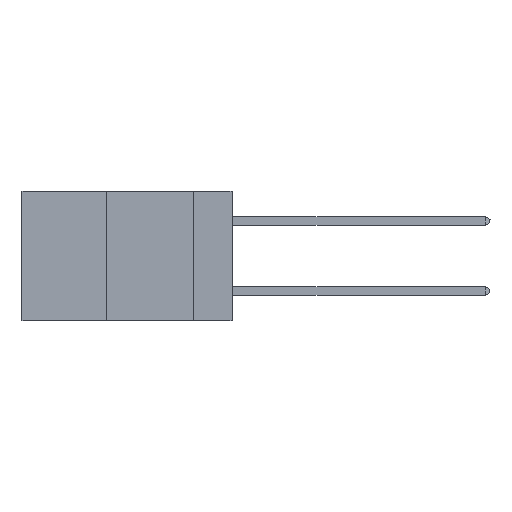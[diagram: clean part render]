
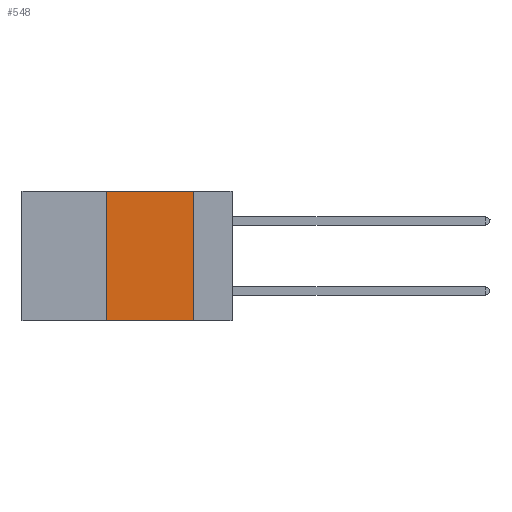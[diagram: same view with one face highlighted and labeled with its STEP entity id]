
A CAD part, left-side view. The second image highlights one B-rep face of the part: STEP entity #548.
In plain terms, the highlighted planar face has unit normal (-1, 0, 0).
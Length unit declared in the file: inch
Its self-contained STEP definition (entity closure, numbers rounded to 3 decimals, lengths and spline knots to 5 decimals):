
#548 = ADVANCED_FACE ( 'NONE', ( #35304 ), #9787, .F. ) ;
#2136 = EDGE_CURVE ( 'NONE', #26741, #20578, #5556, .T. ) ;
#3161 = LINE ( 'NONE', #19504, #9393 ) ;
#3196 = CARTESIAN_POINT ( 'NONE',  ( 0., 0.11, -0.37 ) ) ;
#3500 = DIRECTION ( 'NONE',  ( 1., 0., 0. ) ) ;
#3670 = EDGE_CURVE ( 'NONE', #26741, #34960, #12089, .T. ) ;
#5146 = VECTOR ( 'NONE', #12039, 39.37008 ) ;
#5556 = LINE ( 'NONE', #5956, #5146 ) ;
#5815 = VERTEX_POINT ( 'NONE', #9060 ) ;
#5956 = CARTESIAN_POINT ( 'NONE',  ( 0., 0.6, -0.37 ) ) ;
#8514 = CARTESIAN_POINT ( 'NONE',  ( 0., 0.36, -0.37 ) ) ;
#9060 = CARTESIAN_POINT ( 'NONE',  ( 0., 0.11, 0. ) ) ;
#9393 = VECTOR ( 'NONE', #9865, 39.37008 ) ;
#9787 = PLANE ( 'NONE',  #27102 ) ;
#9865 = DIRECTION ( 'NONE',  ( 0., 0., -1. ) ) ;
#12039 = DIRECTION ( 'NONE',  ( 0., -1., 0. ) ) ;
#12089 = LINE ( 'NONE', #24851, #16658 ) ;
#12625 = ORIENTED_EDGE ( 'NONE', *, *, #39955, .F. ) ;
#15103 = LINE ( 'NONE', #33535, #15465 ) ;
#15465 = VECTOR ( 'NONE', #27244, 39.37008 ) ;
#16658 = VECTOR ( 'NONE', #34681, 39.37008 ) ;
#17616 = ORIENTED_EDGE ( 'NONE', *, *, #2136, .T. ) ;
#18419 = EDGE_CURVE ( 'NONE', #34960, #5815, #15103, .T. ) ;
#19504 = CARTESIAN_POINT ( 'NONE',  ( 0., 0.11, 0. ) ) ;
#20578 = VERTEX_POINT ( 'NONE', #3196 ) ;
#20792 = DIRECTION ( 'NONE',  ( 0., 0., -1. ) ) ;
#23921 = CARTESIAN_POINT ( 'NONE',  ( 0., 0.6, 0. ) ) ;
#24851 = CARTESIAN_POINT ( 'NONE',  ( 0., 0.36, 0. ) ) ;
#25073 = ORIENTED_EDGE ( 'NONE', *, *, #3670, .F. ) ;
#25897 = EDGE_LOOP ( 'NONE', ( #12625, #30933, #25073, #17616 ) ) ;
#26741 = VERTEX_POINT ( 'NONE', #8514 ) ;
#27102 = AXIS2_PLACEMENT_3D ( 'NONE', #23921, #3500, #20792 ) ;
#27244 = DIRECTION ( 'NONE',  ( 0., -1., 0. ) ) ;
#29926 = CARTESIAN_POINT ( 'NONE',  ( 0., 0.36, 0. ) ) ;
#30933 = ORIENTED_EDGE ( 'NONE', *, *, #18419, .F. ) ;
#33535 = CARTESIAN_POINT ( 'NONE',  ( 0., 0.6, 0. ) ) ;
#34681 = DIRECTION ( 'NONE',  ( 0., 0., 1. ) ) ;
#34960 = VERTEX_POINT ( 'NONE', #29926 ) ;
#35304 = FACE_OUTER_BOUND ( 'NONE', #25897, .T. ) ;
#39955 = EDGE_CURVE ( 'NONE', #5815, #20578, #3161, .T. ) ;
